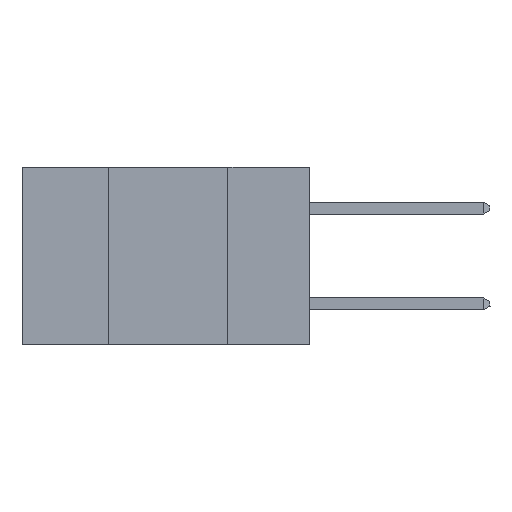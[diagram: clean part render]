
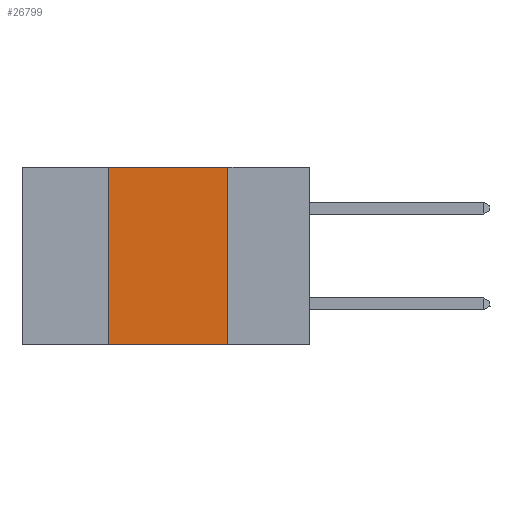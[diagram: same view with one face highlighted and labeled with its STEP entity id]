
A CAD part, left-side view. The second image highlights one B-rep face of the part: STEP entity #26799.
In plain terms, the highlighted planar face has unit normal (-1, 0, 0).
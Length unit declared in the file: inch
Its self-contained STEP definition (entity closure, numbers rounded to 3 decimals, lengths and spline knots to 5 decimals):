
#175 = LINE ( 'NONE', #1488, #26300 ) ;
#182 = ORIENTED_EDGE ( 'NONE', *, *, #28050, .F. ) ;
#857 = CARTESIAN_POINT ( 'NONE',  ( 0., 0.6, 0. ) ) ;
#1488 = CARTESIAN_POINT ( 'NONE',  ( 0., 0.42, 0. ) ) ;
#1714 = EDGE_LOOP ( 'NONE', ( #9336, #182, #25386, #17074 ) ) ;
#1763 = VERTEX_POINT ( 'NONE', #23524 ) ;
#4173 = EDGE_CURVE ( 'NONE', #10128, #22280, #175, .T. ) ;
#5897 = FACE_OUTER_BOUND ( 'NONE', #1714, .T. ) ;
#6172 = VECTOR ( 'NONE', #22396, 39.37008 ) ;
#7084 = DIRECTION ( 'NONE',  ( 0., -1., 0. ) ) ;
#8507 = CARTESIAN_POINT ( 'NONE',  ( 0., 0.6, -0.37 ) ) ;
#9099 = VERTEX_POINT ( 'NONE', #20606 ) ;
#9336 = ORIENTED_EDGE ( 'NONE', *, *, #13550, .F. ) ;
#9865 = VECTOR ( 'NONE', #21451, 39.37008 ) ;
#10128 = VERTEX_POINT ( 'NONE', #24955 ) ;
#10411 = CARTESIAN_POINT ( 'NONE',  ( 0., 0.42, 0. ) ) ;
#10958 = CARTESIAN_POINT ( 'NONE',  ( 0., 0.6, 0. ) ) ;
#13550 = EDGE_CURVE ( 'NONE', #9099, #1763, #28578, .T. ) ;
#14755 = AXIS2_PLACEMENT_3D ( 'NONE', #857, #18822, #27955 ) ;
#15320 = LINE ( 'NONE', #10958, #23796 ) ;
#17074 = ORIENTED_EDGE ( 'NONE', *, *, #17659, .T. ) ;
#17659 = EDGE_CURVE ( 'NONE', #10128, #1763, #22733, .T. ) ;
#18822 = DIRECTION ( 'NONE',  ( 1., 0., 0. ) ) ;
#20606 = CARTESIAN_POINT ( 'NONE',  ( 0., 0.17, 0. ) ) ;
#21451 = DIRECTION ( 'NONE',  ( 0., 0., -1. ) ) ;
#22280 = VERTEX_POINT ( 'NONE', #10411 ) ;
#22396 = DIRECTION ( 'NONE',  ( 0., -1., 0. ) ) ;
#22733 = LINE ( 'NONE', #8507, #6172 ) ;
#23524 = CARTESIAN_POINT ( 'NONE',  ( 0., 0.17, -0.37 ) ) ;
#23796 = VECTOR ( 'NONE', #7084, 39.37008 ) ;
#24955 = CARTESIAN_POINT ( 'NONE',  ( 0., 0.42, -0.37 ) ) ;
#25386 = ORIENTED_EDGE ( 'NONE', *, *, #4173, .F. ) ;
#25695 = PLANE ( 'NONE',  #14755 ) ;
#26187 = CARTESIAN_POINT ( 'NONE',  ( 0., 0.17, 0. ) ) ;
#26300 = VECTOR ( 'NONE', #28867, 39.37008 ) ;
#26799 = ADVANCED_FACE ( 'NONE', ( #5897 ), #25695, .F. ) ;
#27955 = DIRECTION ( 'NONE',  ( 0., 0., -1. ) ) ;
#28050 = EDGE_CURVE ( 'NONE', #22280, #9099, #15320, .T. ) ;
#28578 = LINE ( 'NONE', #26187, #9865 ) ;
#28867 = DIRECTION ( 'NONE',  ( 0., 0., 1. ) ) ;
